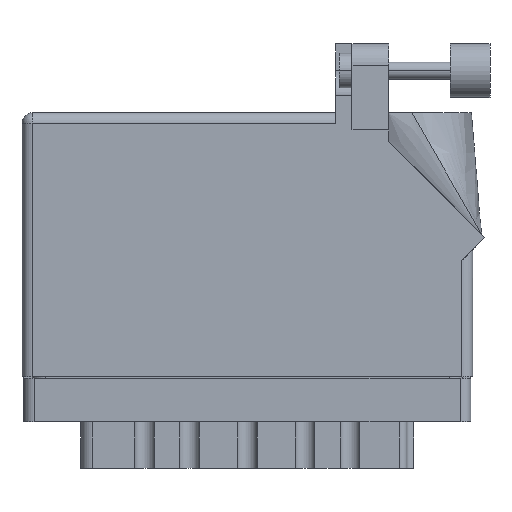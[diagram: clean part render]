
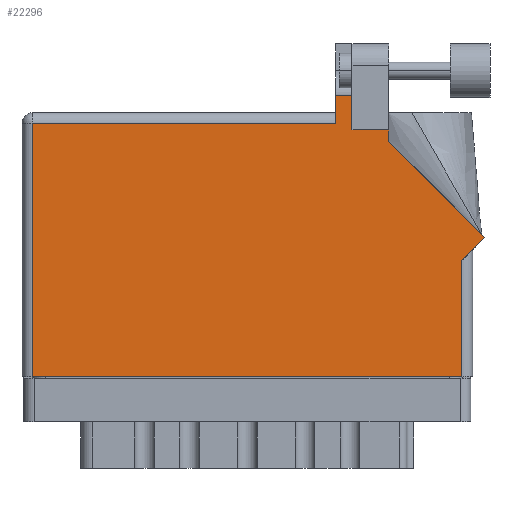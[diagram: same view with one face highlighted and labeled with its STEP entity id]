
A CAD part, front view. The second image highlights one B-rep face of the part: STEP entity #22296.
In plain terms, the highlighted face is planar.
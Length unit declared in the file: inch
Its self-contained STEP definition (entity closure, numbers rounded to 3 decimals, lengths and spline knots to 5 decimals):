
#688 = EDGE_CURVE ( 'NONE', #16687, #40285, #22511, .T. ) ;
#2219 = CARTESIAN_POINT ( 'NONE',  ( 1.819, 1.53, 0. ) ) ;
#2512 = CARTESIAN_POINT ( 'NONE',  ( 2.126, 1.43, 0. ) ) ;
#3624 = LINE ( 'NONE', #30122, #34888 ) ;
#3905 = ORIENTED_EDGE ( 'NONE', *, *, #22994, .T. ) ;
#4495 = VERTEX_POINT ( 'NONE', #13663 ) ;
#6244 = DIRECTION ( 'NONE',  ( 0., 1., 0. ) ) ;
#6469 = PLANE ( 'NONE',  #51080 ) ;
#6992 = CARTESIAN_POINT ( 'NONE',  ( 0., 0., 0. ) ) ;
#7116 = CARTESIAN_POINT ( 'NONE',  ( 2.126, 1.43, 0. ) ) ;
#7187 = CARTESIAN_POINT ( 'NONE',  ( 1.913, 1.43, 0. ) ) ;
#7351 = VERTEX_POINT ( 'NONE', #2512 ) ;
#7452 = VECTOR ( 'NONE', #14703, 39.37008 ) ;
#7487 = LINE ( 'NONE', #24818, #20500 ) ;
#7731 = CARTESIAN_POINT ( 'NONE',  ( 2.126, 1.36442, 0. ) ) ;
#7873 = ORIENTED_EDGE ( 'NONE', *, *, #47266, .T. ) ;
#8108 = DIRECTION ( 'NONE',  ( -1., 0., 0. ) ) ;
#9211 = DIRECTION ( 'NONE',  ( 0., 1., 0. ) ) ;
#9524 = CARTESIAN_POINT ( 'NONE',  ( 2.55, 0.675, 0. ) ) ;
#9624 = LINE ( 'NONE', #7116, #32410 ) ;
#10853 = DIRECTION ( 'NONE',  ( -1., 0., 0. ) ) ;
#11019 = EDGE_CURVE ( 'NONE', #39516, #13286, #16562, .T. ) ;
#11029 = LINE ( 'NONE', #36438, #40335 ) ;
#11551 = CARTESIAN_POINT ( 'NONE',  ( 1.819, 1.468, 0. ) ) ;
#11662 = CARTESIAN_POINT ( 'NONE',  ( 2.68271, 0.80771, 0. ) ) ;
#11735 = CARTESIAN_POINT ( 'NONE',  ( 0.062, 1.468, 0. ) ) ;
#12762 = DIRECTION ( 'NONE',  ( -1., 0., 0. ) ) ;
#13286 = VERTEX_POINT ( 'NONE', #7731 ) ;
#13663 = CARTESIAN_POINT ( 'NONE',  ( 1.913, 1.6315, 0. ) ) ;
#14339 = CARTESIAN_POINT ( 'NONE',  ( 2.68271, 0.80771, 0. ) ) ;
#14422 = VERTEX_POINT ( 'NONE', #28377 ) ;
#14703 = DIRECTION ( 'NONE',  ( -0.707, 0.707, 0. ) ) ;
#14855 = VECTOR ( 'NONE', #48078, 39.37008 ) ;
#16562 = LINE ( 'NONE', #14339, #7452 ) ;
#16687 = VERTEX_POINT ( 'NONE', #47329 ) ;
#17076 = LINE ( 'NONE', #17772, #19680 ) ;
#17121 = VECTOR ( 'NONE', #6244, 39.37008 ) ;
#17438 = VERTEX_POINT ( 'NONE', #11735 ) ;
#17509 = ORIENTED_EDGE ( 'NONE', *, *, #17533, .T. ) ;
#17533 = EDGE_CURVE ( 'NONE', #4495, #21661, #26177, .T. ) ;
#17772 = CARTESIAN_POINT ( 'NONE',  ( 2.55, 0.737, 0. ) ) ;
#19592 = CARTESIAN_POINT ( 'NONE',  ( 0., 1.53, 0. ) ) ;
#19680 = VECTOR ( 'NONE', #9211, 39.37008 ) ;
#20101 = LINE ( 'NONE', #2219, #14855 ) ;
#20500 = VECTOR ( 'NONE', #12762, 39.37008 ) ;
#21661 = VERTEX_POINT ( 'NONE', #21795 ) ;
#21795 = CARTESIAN_POINT ( 'NONE',  ( 1.819, 1.6315, 0. ) ) ;
#22296 = ADVANCED_FACE ( 'NONE', ( #44336 ), #6469, .F. ) ;
#22376 = VERTEX_POINT ( 'NONE', #11551 ) ;
#22511 = LINE ( 'NONE', #6992, #23822 ) ;
#22994 = EDGE_CURVE ( 'NONE', #17438, #16687, #11029, .T. ) ;
#23434 = DIRECTION ( 'NONE',  ( 0., 1., 0. ) ) ;
#23596 = DIRECTION ( 'NONE',  ( 1., 0., 0. ) ) ;
#23822 = VECTOR ( 'NONE', #23596, 39.37008 ) ;
#24217 = EDGE_LOOP ( 'NONE', ( #29233, #17509, #37862, #47899, #3905, #27368, #7873, #35235, #39682, #53004, #47214 ) ) ;
#24818 = CARTESIAN_POINT ( 'NONE',  ( 0., 1.468, 0. ) ) ;
#24933 = EDGE_CURVE ( 'NONE', #14422, #4495, #35565, .T. ) ;
#26177 = LINE ( 'NONE', #41419, #50234 ) ;
#27368 = ORIENTED_EDGE ( 'NONE', *, *, #688, .T. ) ;
#28377 = CARTESIAN_POINT ( 'NONE',  ( 1.913, 1.43, 0. ) ) ;
#29233 = ORIENTED_EDGE ( 'NONE', *, *, #24933, .T. ) ;
#30122 = CARTESIAN_POINT ( 'NONE',  ( 2.612, 0.737, 0. ) ) ;
#31412 = DIRECTION ( 'NONE',  ( 0., 0., -1. ) ) ;
#31416 = LINE ( 'NONE', #35359, #17121 ) ;
#32410 = VECTOR ( 'NONE', #49175, 39.37008 ) ;
#33430 = EDGE_CURVE ( 'NONE', #22376, #17438, #7487, .T. ) ;
#33507 = VERTEX_POINT ( 'NONE', #9524 ) ;
#34888 = VECTOR ( 'NONE', #37978, 39.37008 ) ;
#34946 = EDGE_CURVE ( 'NONE', #13286, #7351, #31416, .T. ) ;
#35235 = ORIENTED_EDGE ( 'NONE', *, *, #42212, .T. ) ;
#35359 = CARTESIAN_POINT ( 'NONE',  ( 2.126, 1.36442, 0. ) ) ;
#35565 = LINE ( 'NONE', #7187, #44717 ) ;
#36438 = CARTESIAN_POINT ( 'NONE',  ( 0.062, 0., 0. ) ) ;
#37457 = CARTESIAN_POINT ( 'NONE',  ( 2.55, 0., 0. ) ) ;
#37741 = EDGE_CURVE ( 'NONE', #21661, #22376, #20101, .T. ) ;
#37862 = ORIENTED_EDGE ( 'NONE', *, *, #37741, .T. ) ;
#37978 = DIRECTION ( 'NONE',  ( 0.707, 0.707, 0. ) ) ;
#39362 = EDGE_CURVE ( 'NONE', #7351, #14422, #9624, .T. ) ;
#39516 = VERTEX_POINT ( 'NONE', #11662 ) ;
#39682 = ORIENTED_EDGE ( 'NONE', *, *, #11019, .T. ) ;
#40285 = VERTEX_POINT ( 'NONE', #37457 ) ;
#40335 = VECTOR ( 'NONE', #40440, 39.37008 ) ;
#40440 = DIRECTION ( 'NONE',  ( 0., -1., 0. ) ) ;
#41419 = CARTESIAN_POINT ( 'NONE',  ( 2.24377, 1.6315, 0. ) ) ;
#42212 = EDGE_CURVE ( 'NONE', #33507, #39516, #3624, .T. ) ;
#44336 = FACE_OUTER_BOUND ( 'NONE', #24217, .T. ) ;
#44717 = VECTOR ( 'NONE', #23434, 39.37008 ) ;
#47214 = ORIENTED_EDGE ( 'NONE', *, *, #39362, .T. ) ;
#47266 = EDGE_CURVE ( 'NONE', #40285, #33507, #17076, .T. ) ;
#47329 = CARTESIAN_POINT ( 'NONE',  ( 0.062, 0., 0. ) ) ;
#47899 = ORIENTED_EDGE ( 'NONE', *, *, #33430, .T. ) ;
#48078 = DIRECTION ( 'NONE',  ( 0., -1., 0. ) ) ;
#49175 = DIRECTION ( 'NONE',  ( -1., 0., 0. ) ) ;
#50234 = VECTOR ( 'NONE', #8108, 39.37008 ) ;
#51080 = AXIS2_PLACEMENT_3D ( 'NONE', #19592, #31412, #10853 ) ;
#53004 = ORIENTED_EDGE ( 'NONE', *, *, #34946, .T. ) ;
